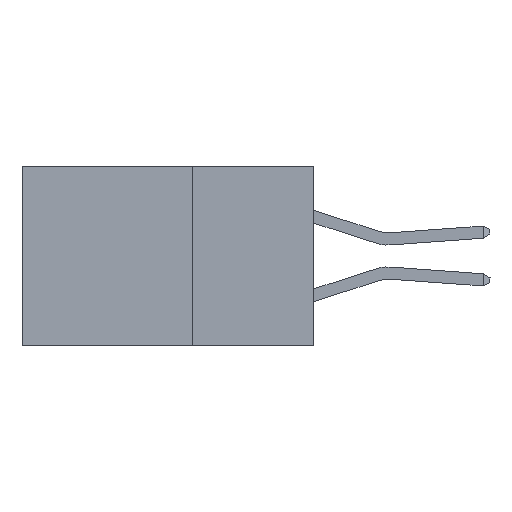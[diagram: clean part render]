
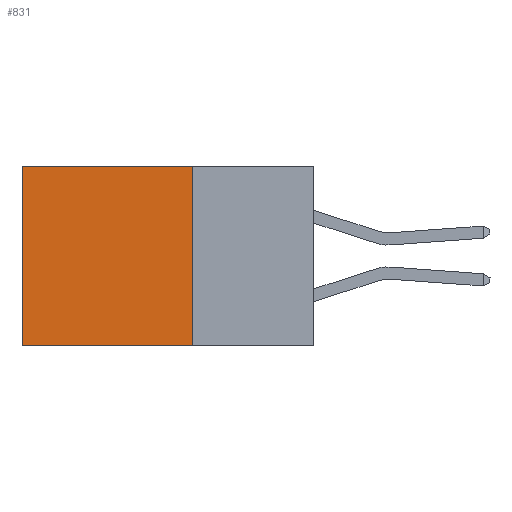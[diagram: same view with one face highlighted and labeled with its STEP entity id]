
A CAD part, left-side view. The second image highlights one B-rep face of the part: STEP entity #831.
In plain terms, the highlighted planar face has unit normal (-1, 0, 0).
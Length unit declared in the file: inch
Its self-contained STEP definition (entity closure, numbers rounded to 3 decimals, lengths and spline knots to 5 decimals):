
#26 = VECTOR ( 'NONE', #3423, 39.37008 ) ;
#694 = CARTESIAN_POINT ( 'NONE',  ( 0.2875, 0.6, -0.37 ) ) ;
#705 = VERTEX_POINT ( 'NONE', #8254 ) ;
#831 = ADVANCED_FACE ( 'NONE', ( #10229 ), #9151, .F. ) ;
#1055 = VECTOR ( 'NONE', #10403, 39.37008 ) ;
#1425 = VECTOR ( 'NONE', #1971, 39.37008 ) ;
#1971 = DIRECTION ( 'NONE',  ( 0., 1., 0. ) ) ;
#2916 = CARTESIAN_POINT ( 'NONE',  ( 0.2875, 0.25, 0. ) ) ;
#3423 = DIRECTION ( 'NONE',  ( 0., 0., -1. ) ) ;
#3536 = ORIENTED_EDGE ( 'NONE', *, *, #6811, .F. ) ;
#5269 = CARTESIAN_POINT ( 'NONE',  ( 0.2875, 0.6, 0. ) ) ;
#5724 = LINE ( 'NONE', #6792, #1055 ) ;
#6792 = CARTESIAN_POINT ( 'NONE',  ( 0.2875, 0.25, -0.37 ) ) ;
#6811 = EDGE_CURVE ( 'NONE', #12242, #10962, #5724, .T. ) ;
#6872 = EDGE_LOOP ( 'NONE', ( #10077, #3536, #15254, #13943 ) ) ;
#7210 = CARTESIAN_POINT ( 'NONE',  ( 0.2875, 0.25, 0. ) ) ;
#7231 = EDGE_CURVE ( 'NONE', #14446, #705, #8579, .T. ) ;
#7724 = AXIS2_PLACEMENT_3D ( 'NONE', #2916, #13994, #14158 ) ;
#8124 = EDGE_CURVE ( 'NONE', #14446, #12242, #10276, .T. ) ;
#8180 = VECTOR ( 'NONE', #12460, 39.37008 ) ;
#8254 = CARTESIAN_POINT ( 'NONE',  ( 0.2875, 0.6, 0. ) ) ;
#8579 = LINE ( 'NONE', #9564, #1425 ) ;
#8587 = EDGE_CURVE ( 'NONE', #705, #10962, #10627, .T. ) ;
#9151 = PLANE ( 'NONE',  #7724 ) ;
#9564 = CARTESIAN_POINT ( 'NONE',  ( 0.2875, 0.25, 0. ) ) ;
#9715 = CARTESIAN_POINT ( 'NONE',  ( 0.2875, 0.25, 0. ) ) ;
#10077 = ORIENTED_EDGE ( 'NONE', *, *, #8587, .T. ) ;
#10229 = FACE_OUTER_BOUND ( 'NONE', #6872, .T. ) ;
#10276 = LINE ( 'NONE', #9715, #26 ) ;
#10403 = DIRECTION ( 'NONE',  ( 0., 1., 0. ) ) ;
#10627 = LINE ( 'NONE', #5269, #8180 ) ;
#10962 = VERTEX_POINT ( 'NONE', #694 ) ;
#12242 = VERTEX_POINT ( 'NONE', #12863 ) ;
#12460 = DIRECTION ( 'NONE',  ( 0., 0., -1. ) ) ;
#12863 = CARTESIAN_POINT ( 'NONE',  ( 0.2875, 0.25, -0.37 ) ) ;
#13943 = ORIENTED_EDGE ( 'NONE', *, *, #7231, .T. ) ;
#13994 = DIRECTION ( 'NONE',  ( 1., 0., 0. ) ) ;
#14158 = DIRECTION ( 'NONE',  ( 0., 0., -1. ) ) ;
#14446 = VERTEX_POINT ( 'NONE', #7210 ) ;
#15254 = ORIENTED_EDGE ( 'NONE', *, *, #8124, .F. ) ;
